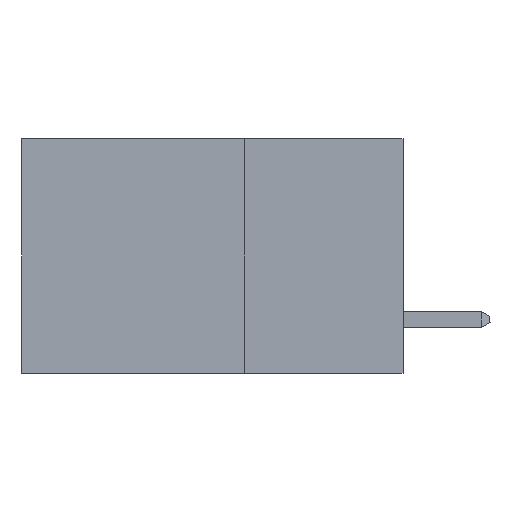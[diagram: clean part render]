
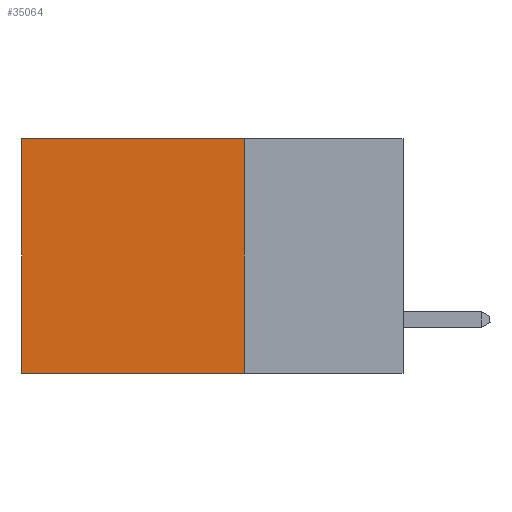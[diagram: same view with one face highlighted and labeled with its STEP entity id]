
A CAD part, left-side view. The second image highlights one B-rep face of the part: STEP entity #35064.
In plain terms, the highlighted planar face has unit normal (-1, 0, 0).
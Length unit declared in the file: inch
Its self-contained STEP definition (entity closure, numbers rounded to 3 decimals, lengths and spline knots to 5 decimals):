
#789 = VECTOR ( 'NONE', #29062, 39.37008 ) ;
#828 = VECTOR ( 'NONE', #6460, 39.37008 ) ;
#920 = EDGE_CURVE ( 'NONE', #10746, #27755, #26488, .T. ) ;
#994 = CARTESIAN_POINT ( 'NONE',  ( 0.2875, 0.25, -0.37 ) ) ;
#1329 = ORIENTED_EDGE ( 'NONE', *, *, #11303, .F. ) ;
#1821 = LINE ( 'NONE', #5661, #789 ) ;
#2681 = ORIENTED_EDGE ( 'NONE', *, *, #15085, .F. ) ;
#3303 = LINE ( 'NONE', #38795, #31074 ) ;
#4343 = AXIS2_PLACEMENT_3D ( 'NONE', #24222, #20986, #17203 ) ;
#5661 = CARTESIAN_POINT ( 'NONE',  ( 0.2875, 0.25, 0. ) ) ;
#6000 = CARTESIAN_POINT ( 'NONE',  ( 0.2875, 0.6, 0. ) ) ;
#6460 = DIRECTION ( 'NONE',  ( 0., 0., -1. ) ) ;
#9178 = VERTEX_POINT ( 'NONE', #12231 ) ;
#9793 = CARTESIAN_POINT ( 'NONE',  ( 0.2875, 0.6, 0. ) ) ;
#10746 = VERTEX_POINT ( 'NONE', #6000 ) ;
#11303 = EDGE_CURVE ( 'NONE', #9178, #40840, #1821, .T. ) ;
#12231 = CARTESIAN_POINT ( 'NONE',  ( 0.2875, 0.25, 0. ) ) ;
#15085 = EDGE_CURVE ( 'NONE', #40840, #27755, #39556, .T. ) ;
#15846 = DIRECTION ( 'NONE',  ( 0., 1., 0. ) ) ;
#17203 = DIRECTION ( 'NONE',  ( 0., 0., -1. ) ) ;
#18924 = FACE_OUTER_BOUND ( 'NONE', #33571, .T. ) ;
#20986 = DIRECTION ( 'NONE',  ( 1., 0., 0. ) ) ;
#22612 = EDGE_CURVE ( 'NONE', #9178, #10746, #3303, .T. ) ;
#24222 = CARTESIAN_POINT ( 'NONE',  ( 0.2875, 0.25, 0. ) ) ;
#25998 = VECTOR ( 'NONE', #33823, 39.37008 ) ;
#26488 = LINE ( 'NONE', #9793, #828 ) ;
#26719 = CARTESIAN_POINT ( 'NONE',  ( 0.2875, 0.25, -0.37 ) ) ;
#27178 = PLANE ( 'NONE',  #4343 ) ;
#27755 = VERTEX_POINT ( 'NONE', #38306 ) ;
#29062 = DIRECTION ( 'NONE',  ( 0., 0., -1. ) ) ;
#31074 = VECTOR ( 'NONE', #15846, 39.37008 ) ;
#32087 = ORIENTED_EDGE ( 'NONE', *, *, #22612, .T. ) ;
#33571 = EDGE_LOOP ( 'NONE', ( #37743, #2681, #1329, #32087 ) ) ;
#33823 = DIRECTION ( 'NONE',  ( 0., 1., 0. ) ) ;
#35064 = ADVANCED_FACE ( 'NONE', ( #18924 ), #27178, .F. ) ;
#37743 = ORIENTED_EDGE ( 'NONE', *, *, #920, .T. ) ;
#38306 = CARTESIAN_POINT ( 'NONE',  ( 0.2875, 0.6, -0.37 ) ) ;
#38795 = CARTESIAN_POINT ( 'NONE',  ( 0.2875, 0.25, 0. ) ) ;
#39556 = LINE ( 'NONE', #26719, #25998 ) ;
#40840 = VERTEX_POINT ( 'NONE', #994 ) ;
